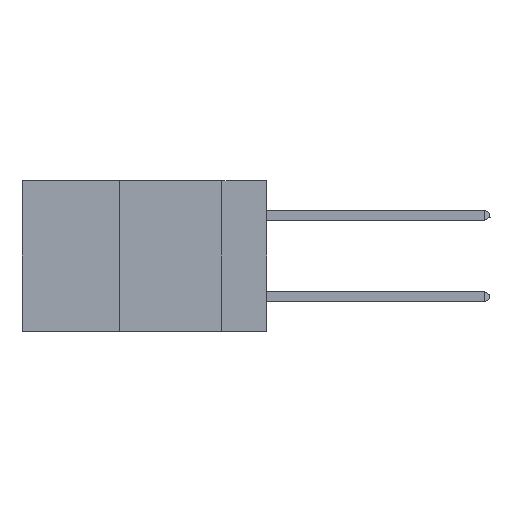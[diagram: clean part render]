
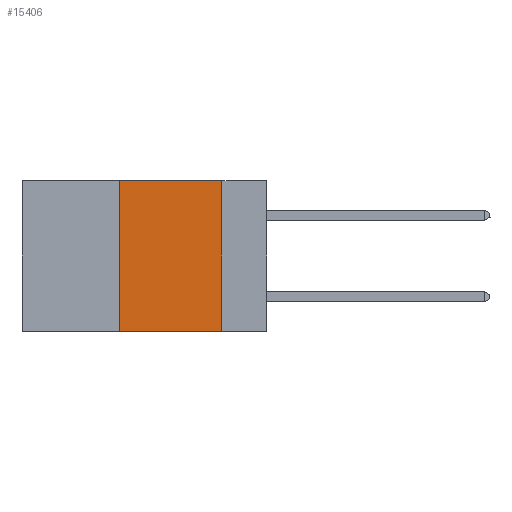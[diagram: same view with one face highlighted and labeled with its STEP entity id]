
A CAD part, left-side view. The second image highlights one B-rep face of the part: STEP entity #15406.
In plain terms, the highlighted planar face has unit normal (-1, 0, 0).
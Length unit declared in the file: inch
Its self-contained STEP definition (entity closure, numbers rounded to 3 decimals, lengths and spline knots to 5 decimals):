
#59 = EDGE_CURVE ( 'NONE', #13531, #20341, #445, .T. ) ;
#208 = LINE ( 'NONE', #16624, #7426 ) ;
#445 = LINE ( 'NONE', #19095, #13610 ) ;
#777 = LINE ( 'NONE', #8987, #1578 ) ;
#1578 = VECTOR ( 'NONE', #9499, 39.37008 ) ;
#3237 = ORIENTED_EDGE ( 'NONE', *, *, #12353, .T. ) ;
#3763 = ORIENTED_EDGE ( 'NONE', *, *, #59, .F. ) ;
#4005 = CARTESIAN_POINT ( 'NONE',  ( 0., 0.11, 0. ) ) ;
#6405 = CARTESIAN_POINT ( 'NONE',  ( 0., 0.6, 0. ) ) ;
#7424 = VERTEX_POINT ( 'NONE', #9367 ) ;
#7426 = VECTOR ( 'NONE', #13649, 39.37008 ) ;
#7855 = FACE_OUTER_BOUND ( 'NONE', #10945, .T. ) ;
#7942 = CARTESIAN_POINT ( 'NONE',  ( 0., 0.11, 0. ) ) ;
#8247 = EDGE_CURVE ( 'NONE', #16105, #13531, #208, .T. ) ;
#8607 = LINE ( 'NONE', #7942, #10649 ) ;
#8987 = CARTESIAN_POINT ( 'NONE',  ( 0., 0.6, -0.37 ) ) ;
#9367 = CARTESIAN_POINT ( 'NONE',  ( 0., 0.11, -0.37 ) ) ;
#9398 = AXIS2_PLACEMENT_3D ( 'NONE', #6405, #17885, #10045 ) ;
#9499 = DIRECTION ( 'NONE',  ( 0., -1., 0. ) ) ;
#10045 = DIRECTION ( 'NONE',  ( 0., 0., -1. ) ) ;
#10649 = VECTOR ( 'NONE', #10791, 39.37008 ) ;
#10791 = DIRECTION ( 'NONE',  ( 0., 0., -1. ) ) ;
#10945 = EDGE_LOOP ( 'NONE', ( #13836, #3763, #15308, #3237 ) ) ;
#12353 = EDGE_CURVE ( 'NONE', #16105, #7424, #777, .T. ) ;
#13156 = PLANE ( 'NONE',  #9398 ) ;
#13531 = VERTEX_POINT ( 'NONE', #13570 ) ;
#13570 = CARTESIAN_POINT ( 'NONE',  ( 0., 0.36, 0. ) ) ;
#13610 = VECTOR ( 'NONE', #19019, 39.37008 ) ;
#13649 = DIRECTION ( 'NONE',  ( 0., 0., 1. ) ) ;
#13836 = ORIENTED_EDGE ( 'NONE', *, *, #19488, .F. ) ;
#15308 = ORIENTED_EDGE ( 'NONE', *, *, #8247, .F. ) ;
#15406 = ADVANCED_FACE ( 'NONE', ( #7855 ), #13156, .F. ) ;
#16105 = VERTEX_POINT ( 'NONE', #18560 ) ;
#16624 = CARTESIAN_POINT ( 'NONE',  ( 0., 0.36, 0. ) ) ;
#17885 = DIRECTION ( 'NONE',  ( 1., 0., 0. ) ) ;
#18560 = CARTESIAN_POINT ( 'NONE',  ( 0., 0.36, -0.37 ) ) ;
#19019 = DIRECTION ( 'NONE',  ( 0., -1., 0. ) ) ;
#19095 = CARTESIAN_POINT ( 'NONE',  ( 0., 0.6, 0. ) ) ;
#19488 = EDGE_CURVE ( 'NONE', #20341, #7424, #8607, .T. ) ;
#20341 = VERTEX_POINT ( 'NONE', #4005 ) ;
